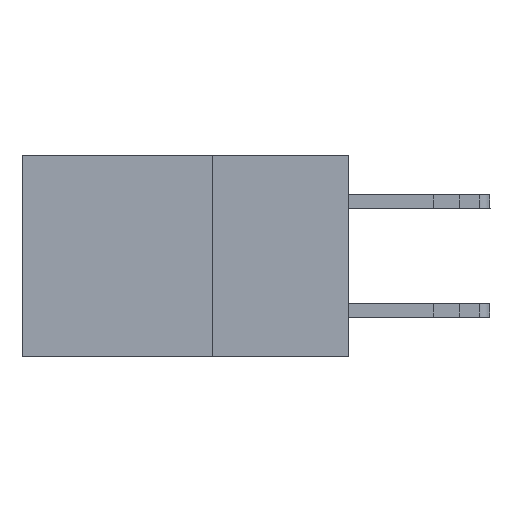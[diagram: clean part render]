
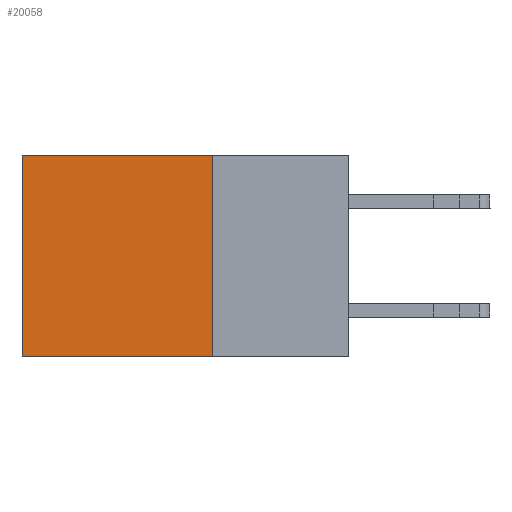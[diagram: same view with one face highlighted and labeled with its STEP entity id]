
A CAD part, left-side view. The second image highlights one B-rep face of the part: STEP entity #20058.
In plain terms, the highlighted planar face has unit normal (-1, 0, 0).
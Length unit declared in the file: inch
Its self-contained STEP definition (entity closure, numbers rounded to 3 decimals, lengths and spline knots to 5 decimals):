
#509 = EDGE_CURVE ( 'NONE', #2022, #5215, #4421, .T. ) ;
#1637 = EDGE_CURVE ( 'NONE', #11331, #2022, #6917, .T. ) ;
#1651 = VERTEX_POINT ( 'NONE', #2757 ) ;
#2022 = VERTEX_POINT ( 'NONE', #11310 ) ;
#2757 = CARTESIAN_POINT ( 'NONE',  ( 0.2615, 0.6, 0. ) ) ;
#4421 = LINE ( 'NONE', #15123, #8612 ) ;
#4471 = ORIENTED_EDGE ( 'NONE', *, *, #17249, .T. ) ;
#5215 = VERTEX_POINT ( 'NONE', #17762 ) ;
#6917 = LINE ( 'NONE', #14383, #20036 ) ;
#7495 = CARTESIAN_POINT ( 'NONE',  ( 0.2615, 0.25, 0. ) ) ;
#7546 = DIRECTION ( 'NONE',  ( 0., 1., 0. ) ) ;
#7655 = ORIENTED_EDGE ( 'NONE', *, *, #8888, .T. ) ;
#7848 = PLANE ( 'NONE',  #10031 ) ;
#8235 = EDGE_LOOP ( 'NONE', ( #4471, #9657, #12462, #7655 ) ) ;
#8612 = VECTOR ( 'NONE', #10413, 39.37008 ) ;
#8888 = EDGE_CURVE ( 'NONE', #11331, #1651, #17806, .T. ) ;
#9605 = DIRECTION ( 'NONE',  ( 0., 0., -1. ) ) ;
#9657 = ORIENTED_EDGE ( 'NONE', *, *, #509, .F. ) ;
#10031 = AXIS2_PLACEMENT_3D ( 'NONE', #14680, #19767, #9605 ) ;
#10354 = CARTESIAN_POINT ( 'NONE',  ( 0.2615, 0.25, 0. ) ) ;
#10413 = DIRECTION ( 'NONE',  ( 0., 1., 0. ) ) ;
#10783 = FACE_OUTER_BOUND ( 'NONE', #8235, .T. ) ;
#10912 = DIRECTION ( 'NONE',  ( 0., 0., -1. ) ) ;
#11310 = CARTESIAN_POINT ( 'NONE',  ( 0.2615, 0.25, -0.37 ) ) ;
#11331 = VERTEX_POINT ( 'NONE', #10354 ) ;
#12462 = ORIENTED_EDGE ( 'NONE', *, *, #1637, .F. ) ;
#13001 = VECTOR ( 'NONE', #10912, 39.37008 ) ;
#14383 = CARTESIAN_POINT ( 'NONE',  ( 0.2615, 0.25, -0.37 ) ) ;
#14680 = CARTESIAN_POINT ( 'NONE',  ( 0.2615, 0.25, -0.37 ) ) ;
#15123 = CARTESIAN_POINT ( 'NONE',  ( 0.2615, 0.25, -0.37 ) ) ;
#17249 = EDGE_CURVE ( 'NONE', #1651, #5215, #21972, .T. ) ;
#17762 = CARTESIAN_POINT ( 'NONE',  ( 0.2615, 0.6, -0.37 ) ) ;
#17806 = LINE ( 'NONE', #7495, #21206 ) ;
#19353 = CARTESIAN_POINT ( 'NONE',  ( 0.2615, 0.6, -0.37 ) ) ;
#19767 = DIRECTION ( 'NONE',  ( 1., 0., 0. ) ) ;
#20036 = VECTOR ( 'NONE', #21178, 39.37008 ) ;
#20058 = ADVANCED_FACE ( 'NONE', ( #10783 ), #7848, .F. ) ;
#21178 = DIRECTION ( 'NONE',  ( 0., 0., -1. ) ) ;
#21206 = VECTOR ( 'NONE', #7546, 39.37008 ) ;
#21972 = LINE ( 'NONE', #19353, #13001 ) ;
